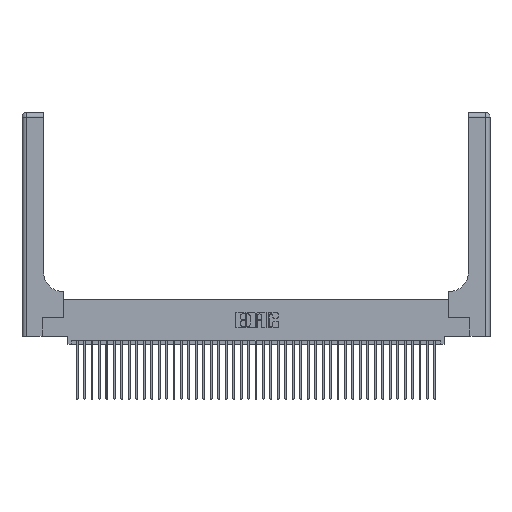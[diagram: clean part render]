
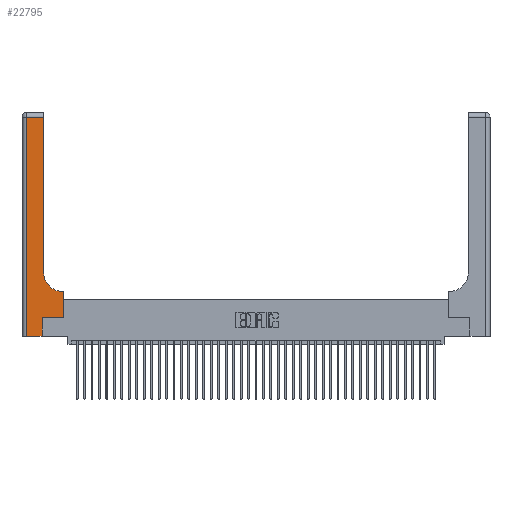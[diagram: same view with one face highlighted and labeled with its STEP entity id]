
A CAD part, top view. The second image highlights one B-rep face of the part: STEP entity #22795.
In plain terms, the highlighted planar face has unit normal (0, 0, 1).
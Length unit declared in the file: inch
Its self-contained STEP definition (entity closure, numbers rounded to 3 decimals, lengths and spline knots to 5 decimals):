
#33 = VERTEX_POINT ( 'NONE', #28741 ) ;
#40 = EDGE_CURVE ( 'NONE', #25767, #15886, #11517, .T. ) ;
#674 = VECTOR ( 'NONE', #35706, 39.37008 ) ;
#780 = VECTOR ( 'NONE', #6082, 39.37008 ) ;
#860 = ORIENTED_EDGE ( 'NONE', *, *, #8331, .T. ) ;
#1430 = LINE ( 'NONE', #28451, #11790 ) ;
#1524 = CARTESIAN_POINT ( 'NONE',  ( 0.5415, 0.6, 0.37 ) ) ;
#1555 = EDGE_CURVE ( 'NONE', #27511, #8418, #29056, .T. ) ;
#1647 = ORIENTED_EDGE ( 'NONE', *, *, #1555, .T. ) ;
#1951 = EDGE_LOOP ( 'NONE', ( #18537, #39405, #11908, #40137, #1647, #6494, #860, #29888, #21951 ) ) ;
#2112 = DIRECTION ( 'NONE',  ( -1., 0., 0. ) ) ;
#2607 = VERTEX_POINT ( 'NONE', #18043 ) ;
#2958 = LINE ( 'NONE', #37777, #10673 ) ;
#4072 = CARTESIAN_POINT ( 'NONE',  ( 0.5585, 0.25, 0.37 ) ) ;
#5261 = CARTESIAN_POINT ( 'NONE',  ( 0., 3., 0.37 ) ) ;
#5351 = DIRECTION ( 'NONE',  ( 0., 1., 0. ) ) ;
#6082 = DIRECTION ( 'NONE',  ( 0., 1., 0. ) ) ;
#6494 = ORIENTED_EDGE ( 'NONE', *, *, #27098, .T. ) ;
#6915 = LINE ( 'NONE', #25484, #674 ) ;
#6971 = LINE ( 'NONE', #22383, #11092 ) ;
#7256 = VECTOR ( 'NONE', #32056, 39.37008 ) ;
#7307 = FACE_OUTER_BOUND ( 'NONE', #1951, .T. ) ;
#8331 = EDGE_CURVE ( 'NONE', #26888, #32694, #19988, .T. ) ;
#8418 = VERTEX_POINT ( 'NONE', #28804 ) ;
#9340 = DIRECTION ( 'NONE',  ( 0., -1., 0. ) ) ;
#10673 = VECTOR ( 'NONE', #5351, 39.37008 ) ;
#11033 = DIRECTION ( 'NONE',  ( 0., 0., -1. ) ) ;
#11092 = VECTOR ( 'NONE', #9340, 39.37008 ) ;
#11517 = CIRCLE ( 'NONE', #38124, 0.25 ) ;
#11790 = VECTOR ( 'NONE', #38258, 39.37008 ) ;
#11908 = ORIENTED_EDGE ( 'NONE', *, *, #35424, .T. ) ;
#13392 = VECTOR ( 'NONE', #15610, 39.37008 ) ;
#15349 = DIRECTION ( 'NONE',  ( 0., 0., -1. ) ) ;
#15369 = EDGE_CURVE ( 'NONE', #33230, #27511, #29506, .T. ) ;
#15610 = DIRECTION ( 'NONE',  ( 1., 0., 0. ) ) ;
#15886 = VERTEX_POINT ( 'NONE', #18079 ) ;
#17085 = EDGE_CURVE ( 'NONE', #15886, #2607, #2958, .T. ) ;
#18043 = CARTESIAN_POINT ( 'NONE',  ( 0.2915, 2.94, 0.37 ) ) ;
#18079 = CARTESIAN_POINT ( 'NONE',  ( 0.2915, 0.85, 0.37 ) ) ;
#18129 = CARTESIAN_POINT ( 'NONE',  ( 0.5415, 0.85, 0.37 ) ) ;
#18537 = ORIENTED_EDGE ( 'NONE', *, *, #17085, .T. ) ;
#19953 = CARTESIAN_POINT ( 'NONE',  ( 0.2915, 0.6, 0.37 ) ) ;
#19988 = LINE ( 'NONE', #32405, #780 ) ;
#20796 = DIRECTION ( 'NONE',  ( -1., 0., 0. ) ) ;
#21951 = ORIENTED_EDGE ( 'NONE', *, *, #40, .T. ) ;
#22383 = CARTESIAN_POINT ( 'NONE',  ( 0.06, 3., 0.37 ) ) ;
#22795 = ADVANCED_FACE ( 'NONE', ( #7307 ), #34902, .F. ) ;
#24546 = EDGE_CURVE ( 'NONE', #32694, #25767, #38718, .T. ) ;
#25370 = DIRECTION ( 'NONE',  ( 1., 0., 0. ) ) ;
#25484 = CARTESIAN_POINT ( 'NONE',  ( 0.269, 0.25, 0.37 ) ) ;
#25492 = AXIS2_PLACEMENT_3D ( 'NONE', #5261, #15349, #2112 ) ;
#25767 = VERTEX_POINT ( 'NONE', #1524 ) ;
#26888 = VERTEX_POINT ( 'NONE', #4072 ) ;
#27098 = EDGE_CURVE ( 'NONE', #8418, #26888, #6915, .T. ) ;
#27511 = VERTEX_POINT ( 'NONE', #27614 ) ;
#27614 = CARTESIAN_POINT ( 'NONE',  ( 0.269, 0., 0.37 ) ) ;
#28451 = CARTESIAN_POINT ( 'NONE',  ( 0., 2.94, 0.37 ) ) ;
#28474 = CARTESIAN_POINT ( 'NONE',  ( 0.269, 0., 0.37 ) ) ;
#28741 = CARTESIAN_POINT ( 'NONE',  ( 0.06, 2.94, 0.37 ) ) ;
#28804 = CARTESIAN_POINT ( 'NONE',  ( 0.269, 0.25, 0.37 ) ) ;
#29056 = LINE ( 'NONE', #28474, #7256 ) ;
#29444 = VECTOR ( 'NONE', #20796, 39.37008 ) ;
#29506 = LINE ( 'NONE', #39387, #13392 ) ;
#29888 = ORIENTED_EDGE ( 'NONE', *, *, #24546, .T. ) ;
#30775 = EDGE_CURVE ( 'NONE', #2607, #33, #1430, .T. ) ;
#32029 = CARTESIAN_POINT ( 'NONE',  ( 0.5585, 0.6, 0.37 ) ) ;
#32056 = DIRECTION ( 'NONE',  ( 0., 1., 0. ) ) ;
#32405 = CARTESIAN_POINT ( 'NONE',  ( 0.5585, 0.25, 0.37 ) ) ;
#32694 = VERTEX_POINT ( 'NONE', #32029 ) ;
#33230 = VERTEX_POINT ( 'NONE', #40377 ) ;
#34902 = PLANE ( 'NONE',  #25492 ) ;
#35424 = EDGE_CURVE ( 'NONE', #33, #33230, #6971, .T. ) ;
#35706 = DIRECTION ( 'NONE',  ( 1., 0., 0. ) ) ;
#37777 = CARTESIAN_POINT ( 'NONE',  ( 0.2915, 3., 0.37 ) ) ;
#38124 = AXIS2_PLACEMENT_3D ( 'NONE', #18129, #11033, #25370 ) ;
#38258 = DIRECTION ( 'NONE',  ( -1., 0., 0. ) ) ;
#38718 = LINE ( 'NONE', #19953, #29444 ) ;
#39387 = CARTESIAN_POINT ( 'NONE',  ( 0., 0., 0.37 ) ) ;
#39405 = ORIENTED_EDGE ( 'NONE', *, *, #30775, .T. ) ;
#40137 = ORIENTED_EDGE ( 'NONE', *, *, #15369, .T. ) ;
#40377 = CARTESIAN_POINT ( 'NONE',  ( 0.06, 0., 0.37 ) ) ;
